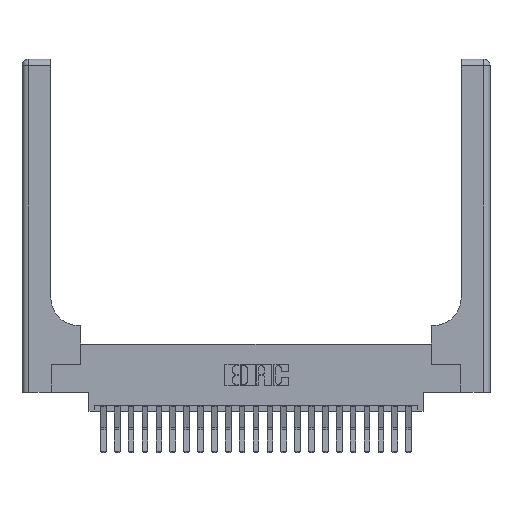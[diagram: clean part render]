
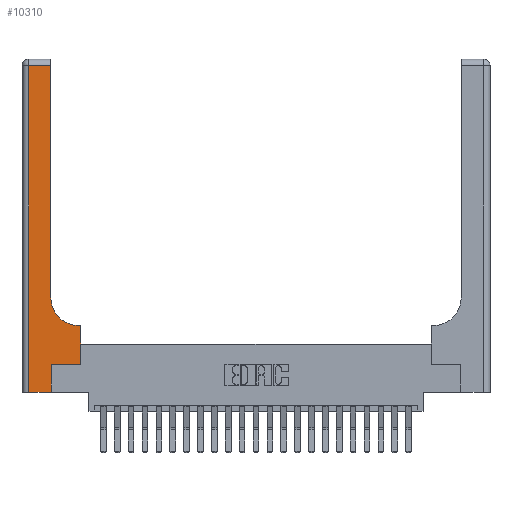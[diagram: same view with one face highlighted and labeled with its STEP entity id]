
A CAD part, top view. The second image highlights one B-rep face of the part: STEP entity #10310.
In plain terms, the highlighted planar face has unit normal (0, 0, 1).
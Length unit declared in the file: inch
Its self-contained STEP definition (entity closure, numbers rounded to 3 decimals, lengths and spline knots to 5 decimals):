
#45 = VERTEX_POINT ( 'NONE', #18247 ) ;
#48 = DIRECTION ( 'NONE',  ( -1., 0., 0. ) ) ;
#198 = ORIENTED_EDGE ( 'NONE', *, *, #8421, .T. ) ;
#292 = FACE_OUTER_BOUND ( 'NONE', #1876, .T. ) ;
#1876 = EDGE_LOOP ( 'NONE', ( #18237, #2964, #198, #11267, #7286, #16685, #13099, #16343, #20631 ) ) ;
#2041 = CARTESIAN_POINT ( 'NONE',  ( 0.265, 0., 0.37 ) ) ;
#2931 = VECTOR ( 'NONE', #11449, 39.37008 ) ;
#2964 = ORIENTED_EDGE ( 'NONE', *, *, #15827, .T. ) ;
#3315 = CARTESIAN_POINT ( 'NONE',  ( 0.06, 0., 0.37 ) ) ;
#3412 = DIRECTION ( 'NONE',  ( 1., 0., 0. ) ) ;
#4291 = VERTEX_POINT ( 'NONE', #15698 ) ;
#4492 = EDGE_CURVE ( 'NONE', #21878, #4291, #20966, .T. ) ;
#4876 = AXIS2_PLACEMENT_3D ( 'NONE', #15729, #5089, #17492 ) ;
#4957 = EDGE_CURVE ( 'NONE', #22848, #21878, #12195, .T. ) ;
#5089 = DIRECTION ( 'NONE',  ( 0., 0., -1. ) ) ;
#5466 = CARTESIAN_POINT ( 'NONE',  ( 0., 2.94, 0.37 ) ) ;
#5544 = EDGE_CURVE ( 'NONE', #19969, #21950, #16048, .T. ) ;
#6006 = LINE ( 'NONE', #5466, #10226 ) ;
#6122 = CARTESIAN_POINT ( 'NONE',  ( 0.26, 3., 0.37 ) ) ;
#6239 = EDGE_CURVE ( 'NONE', #4291, #20202, #17400, .T. ) ;
#6305 = VECTOR ( 'NONE', #12791, 39.37008 ) ;
#6925 = VECTOR ( 'NONE', #16293, 39.37008 ) ;
#7286 = ORIENTED_EDGE ( 'NONE', *, *, #4492, .T. ) ;
#7308 = CARTESIAN_POINT ( 'NONE',  ( 0., 3., 0.37 ) ) ;
#7409 = CARTESIAN_POINT ( 'NONE',  ( 0.06, 3., 0.37 ) ) ;
#8261 = CARTESIAN_POINT ( 'NONE',  ( 0.528, 0.6, 0.37 ) ) ;
#8421 = EDGE_CURVE ( 'NONE', #45, #22848, #13296, .T. ) ;
#9105 = DIRECTION ( 'NONE',  ( 0., 0., -1. ) ) ;
#9587 = CARTESIAN_POINT ( 'NONE',  ( 0.528, 0.25, 0.37 ) ) ;
#9738 = EDGE_CURVE ( 'NONE', #20202, #12148, #20376, .T. ) ;
#9872 = EDGE_CURVE ( 'NONE', #12148, #19969, #17099, .T. ) ;
#10226 = VECTOR ( 'NONE', #48, 39.37008 ) ;
#10310 = ADVANCED_FACE ( 'NONE', ( #292 ), #17894, .F. ) ;
#10357 = CARTESIAN_POINT ( 'NONE',  ( 0., 0., 0.37 ) ) ;
#11267 = ORIENTED_EDGE ( 'NONE', *, *, #4957, .T. ) ;
#11449 = DIRECTION ( 'NONE',  ( -1., 0., 0. ) ) ;
#12148 = VERTEX_POINT ( 'NONE', #8261 ) ;
#12195 = LINE ( 'NONE', #10357, #16863 ) ;
#12791 = DIRECTION ( 'NONE',  ( 0., 1., 0. ) ) ;
#13099 = ORIENTED_EDGE ( 'NONE', *, *, #9738, .T. ) ;
#13296 = LINE ( 'NONE', #7409, #22017 ) ;
#13935 = EDGE_CURVE ( 'NONE', #21950, #18225, #20179, .T. ) ;
#14718 = CARTESIAN_POINT ( 'NONE',  ( 0.265, 0., 0.37 ) ) ;
#15555 = VECTOR ( 'NONE', #20486, 39.37008 ) ;
#15698 = CARTESIAN_POINT ( 'NONE',  ( 0.265, 0.25, 0.37 ) ) ;
#15729 = CARTESIAN_POINT ( 'NONE',  ( 0.51, 0.85, 0.37 ) ) ;
#15827 = EDGE_CURVE ( 'NONE', #18225, #45, #6006, .T. ) ;
#16048 = CIRCLE ( 'NONE', #4876, 0.25 ) ;
#16293 = DIRECTION ( 'NONE',  ( 0., 1., 0. ) ) ;
#16343 = ORIENTED_EDGE ( 'NONE', *, *, #9872, .T. ) ;
#16685 = ORIENTED_EDGE ( 'NONE', *, *, #6239, .T. ) ;
#16840 = VECTOR ( 'NONE', #3412, 39.37008 ) ;
#16863 = VECTOR ( 'NONE', #19130, 39.37008 ) ;
#17099 = LINE ( 'NONE', #20182, #2931 ) ;
#17400 = LINE ( 'NONE', #17535, #16840 ) ;
#17492 = DIRECTION ( 'NONE',  ( 1., 0., 0. ) ) ;
#17535 = CARTESIAN_POINT ( 'NONE',  ( 0.265, 0.25, 0.37 ) ) ;
#17894 = PLANE ( 'NONE',  #22758 ) ;
#18001 = DIRECTION ( 'NONE',  ( 0., -1., 0. ) ) ;
#18225 = VERTEX_POINT ( 'NONE', #19450 ) ;
#18237 = ORIENTED_EDGE ( 'NONE', *, *, #13935, .T. ) ;
#18247 = CARTESIAN_POINT ( 'NONE',  ( 0.06, 2.94, 0.37 ) ) ;
#18541 = CARTESIAN_POINT ( 'NONE',  ( 0.26, 0.85, 0.37 ) ) ;
#19130 = DIRECTION ( 'NONE',  ( 1., 0., 0. ) ) ;
#19450 = CARTESIAN_POINT ( 'NONE',  ( 0.26, 2.94, 0.37 ) ) ;
#19740 = CARTESIAN_POINT ( 'NONE',  ( 0.528, 0.25, 0.37 ) ) ;
#19969 = VERTEX_POINT ( 'NONE', #22764 ) ;
#20179 = LINE ( 'NONE', #6122, #15555 ) ;
#20182 = CARTESIAN_POINT ( 'NONE',  ( 0.26, 0.6, 0.37 ) ) ;
#20202 = VERTEX_POINT ( 'NONE', #9587 ) ;
#20376 = LINE ( 'NONE', #19740, #6305 ) ;
#20486 = DIRECTION ( 'NONE',  ( 0., 1., 0. ) ) ;
#20631 = ORIENTED_EDGE ( 'NONE', *, *, #5544, .T. ) ;
#20966 = LINE ( 'NONE', #2041, #6925 ) ;
#21378 = DIRECTION ( 'NONE',  ( -1., 0., 0. ) ) ;
#21878 = VERTEX_POINT ( 'NONE', #14718 ) ;
#21950 = VERTEX_POINT ( 'NONE', #18541 ) ;
#22017 = VECTOR ( 'NONE', #18001, 39.37008 ) ;
#22758 = AXIS2_PLACEMENT_3D ( 'NONE', #7308, #9105, #21378 ) ;
#22764 = CARTESIAN_POINT ( 'NONE',  ( 0.51, 0.6, 0.37 ) ) ;
#22848 = VERTEX_POINT ( 'NONE', #3315 ) ;
